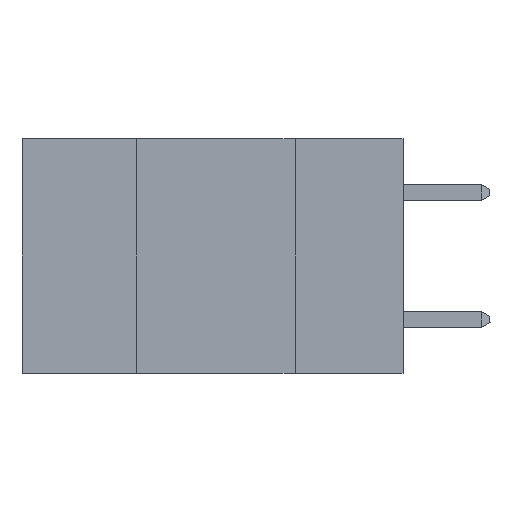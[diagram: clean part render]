
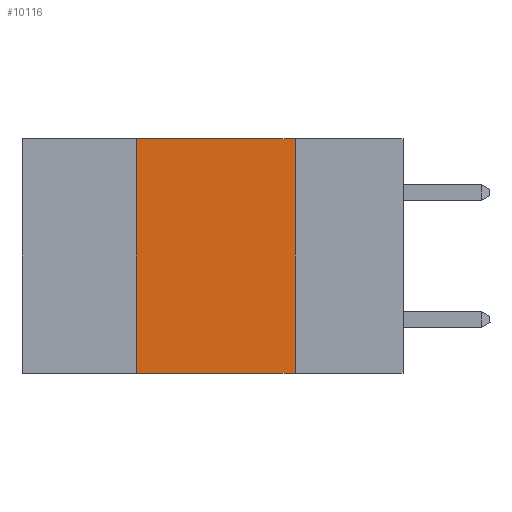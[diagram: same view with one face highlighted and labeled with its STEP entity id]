
A CAD part, left-side view. The second image highlights one B-rep face of the part: STEP entity #10116.
In plain terms, the highlighted planar face has unit normal (-1, 0, 0).
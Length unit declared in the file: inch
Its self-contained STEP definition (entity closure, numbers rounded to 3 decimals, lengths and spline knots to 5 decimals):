
#249 = DIRECTION ( 'NONE',  ( 0., 0., -1. ) ) ;
#434 = CARTESIAN_POINT ( 'NONE',  ( 0., 0.17, 0. ) ) ;
#658 = EDGE_CURVE ( 'NONE', #14366, #12976, #11591, .T. ) ;
#779 = EDGE_LOOP ( 'NONE', ( #2144, #3344, #13141, #14215 ) ) ;
#1206 = EDGE_CURVE ( 'NONE', #12891, #12976, #8099, .T. ) ;
#1726 = VECTOR ( 'NONE', #2087, 39.37008 ) ;
#1998 = CARTESIAN_POINT ( 'NONE',  ( 0., 0.17, 0. ) ) ;
#2011 = VECTOR ( 'NONE', #4343, 39.37008 ) ;
#2087 = DIRECTION ( 'NONE',  ( 0., 0., 1. ) ) ;
#2144 = ORIENTED_EDGE ( 'NONE', *, *, #658, .F. ) ;
#2356 = LINE ( 'NONE', #6243, #14586 ) ;
#2584 = CARTESIAN_POINT ( 'NONE',  ( 0., 0.42, 0. ) ) ;
#3311 = DIRECTION ( 'NONE',  ( 0., -1., 0. ) ) ;
#3344 = ORIENTED_EDGE ( 'NONE', *, *, #15403, .F. ) ;
#3570 = AXIS2_PLACEMENT_3D ( 'NONE', #13449, #7663, #249 ) ;
#4168 = FACE_OUTER_BOUND ( 'NONE', #779, .T. ) ;
#4343 = DIRECTION ( 'NONE',  ( 0., 0., -1. ) ) ;
#4547 = VECTOR ( 'NONE', #3311, 39.37008 ) ;
#4853 = CARTESIAN_POINT ( 'NONE',  ( 0., 0.6, -0.37 ) ) ;
#6129 = VERTEX_POINT ( 'NONE', #2584 ) ;
#6243 = CARTESIAN_POINT ( 'NONE',  ( 0., 0.6, 0. ) ) ;
#6510 = EDGE_CURVE ( 'NONE', #12891, #6129, #11355, .T. ) ;
#7145 = CARTESIAN_POINT ( 'NONE',  ( 0., 0.17, -0.37 ) ) ;
#7663 = DIRECTION ( 'NONE',  ( 1., 0., 0. ) ) ;
#8099 = LINE ( 'NONE', #4853, #4547 ) ;
#9350 = CARTESIAN_POINT ( 'NONE',  ( 0., 0.42, 0. ) ) ;
#9814 = DIRECTION ( 'NONE',  ( 0., -1., 0. ) ) ;
#10116 = ADVANCED_FACE ( 'NONE', ( #4168 ), #14589, .F. ) ;
#11355 = LINE ( 'NONE', #9350, #1726 ) ;
#11591 = LINE ( 'NONE', #1998, #2011 ) ;
#11648 = CARTESIAN_POINT ( 'NONE',  ( 0., 0.42, -0.37 ) ) ;
#12891 = VERTEX_POINT ( 'NONE', #11648 ) ;
#12976 = VERTEX_POINT ( 'NONE', #7145 ) ;
#13141 = ORIENTED_EDGE ( 'NONE', *, *, #6510, .F. ) ;
#13449 = CARTESIAN_POINT ( 'NONE',  ( 0., 0.6, 0. ) ) ;
#14215 = ORIENTED_EDGE ( 'NONE', *, *, #1206, .T. ) ;
#14366 = VERTEX_POINT ( 'NONE', #434 ) ;
#14586 = VECTOR ( 'NONE', #9814, 39.37008 ) ;
#14589 = PLANE ( 'NONE',  #3570 ) ;
#15403 = EDGE_CURVE ( 'NONE', #6129, #14366, #2356, .T. ) ;
